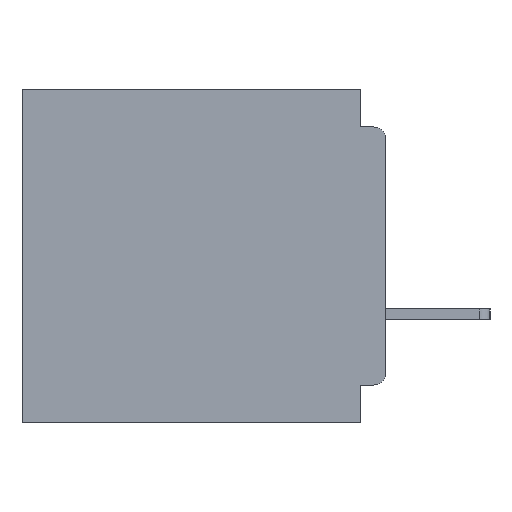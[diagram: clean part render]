
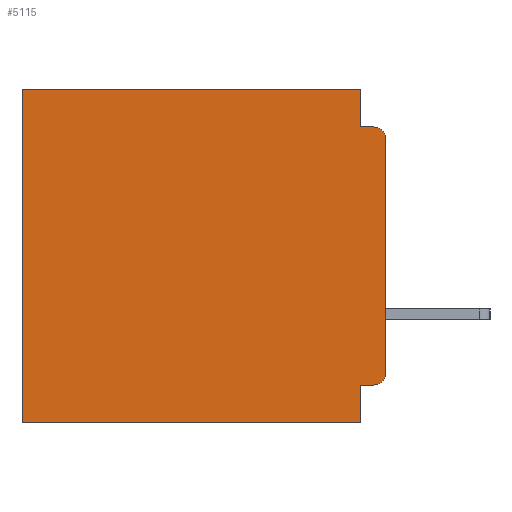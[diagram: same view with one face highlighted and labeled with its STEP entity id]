
A CAD part, left-side view. The second image highlights one B-rep face of the part: STEP entity #5115.
In plain terms, the highlighted planar face has unit normal (-1, 0, 0).
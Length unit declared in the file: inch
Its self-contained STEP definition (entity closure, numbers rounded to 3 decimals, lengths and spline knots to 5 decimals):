
#22 = LINE ( 'NONE', #43585, #37255 ) ;
#1250 = EDGE_CURVE ( 'NONE', #62377, #5661, #42428, .T. ) ;
#1425 = ORIENTED_EDGE ( 'NONE', *, *, #43986, .F. ) ;
#1690 = CARTESIAN_POINT ( 'NONE',  ( 0.3, 0.437, -0.4 ) ) ;
#2197 = CARTESIAN_POINT ( 'NONE',  ( 0.3, 0., -0.4 ) ) ;
#2217 = CARTESIAN_POINT ( 'NONE',  ( 0.3, 0., -0.355 ) ) ;
#5115 = ADVANCED_FACE ( 'NONE', ( #31455 ), #31283, .F. ) ;
#5163 = CIRCLE ( 'NONE', #60748, 0.015 ) ;
#5661 = VERTEX_POINT ( 'NONE', #1690 ) ;
#5747 = CARTESIAN_POINT ( 'NONE',  ( 0.3, 0.015, -0.06 ) ) ;
#5921 = VECTOR ( 'NONE', #22734, 39.37008 ) ;
#5989 = ORIENTED_EDGE ( 'NONE', *, *, #25638, .F. ) ;
#6560 = VERTEX_POINT ( 'NONE', #57812 ) ;
#6705 = DIRECTION ( 'NONE',  ( -1., 0., 0. ) ) ;
#7070 = DIRECTION ( 'NONE',  ( 1., 0., 0. ) ) ;
#9063 = VERTEX_POINT ( 'NONE', #48543 ) ;
#9723 = DIRECTION ( 'NONE',  ( 0., 0., -1. ) ) ;
#9816 = CARTESIAN_POINT ( 'NONE',  ( 0.3, 0.031, -0.4 ) ) ;
#9836 = VERTEX_POINT ( 'NONE', #16102 ) ;
#10659 = DIRECTION ( 'NONE',  ( 0., 0., -1. ) ) ;
#10803 = LINE ( 'NONE', #21135, #36539 ) ;
#12508 = VERTEX_POINT ( 'NONE', #9816 ) ;
#13091 = CARTESIAN_POINT ( 'NONE',  ( 0.3, 0.031, -0.4 ) ) ;
#13799 = LINE ( 'NONE', #33383, #52346 ) ;
#14125 = EDGE_CURVE ( 'NONE', #22895, #6560, #31922, .T. ) ;
#15956 = ORIENTED_EDGE ( 'NONE', *, *, #57442, .F. ) ;
#15957 = CARTESIAN_POINT ( 'NONE',  ( 0.3, 0.031, -0.355 ) ) ;
#16102 = CARTESIAN_POINT ( 'NONE',  ( 0.3, 0.015, -0.355 ) ) ;
#18170 = EDGE_CURVE ( 'NONE', #6560, #48201, #10803, .T. ) ;
#18197 = ORIENTED_EDGE ( 'NONE', *, *, #14125, .F. ) ;
#19009 = CARTESIAN_POINT ( 'NONE',  ( 0.3, 0.031, 0. ) ) ;
#19772 = AXIS2_PLACEMENT_3D ( 'NONE', #2197, #7070, #40961 ) ;
#21135 = CARTESIAN_POINT ( 'NONE',  ( 0.3, 0., -0.045 ) ) ;
#22161 = LINE ( 'NONE', #2217, #46366 ) ;
#22734 = DIRECTION ( 'NONE',  ( 0., 1., 0. ) ) ;
#22895 = VERTEX_POINT ( 'NONE', #56652 ) ;
#23789 = CARTESIAN_POINT ( 'NONE',  ( 0.3, 0.437, -0.4 ) ) ;
#24205 = ORIENTED_EDGE ( 'NONE', *, *, #62770, .F. ) ;
#25397 = VERTEX_POINT ( 'NONE', #54737 ) ;
#25561 = AXIS2_PLACEMENT_3D ( 'NONE', #35741, #6705, #40599 ) ;
#25638 = EDGE_CURVE ( 'NONE', #58649, #12508, #27592, .T. ) ;
#27592 = LINE ( 'NONE', #13091, #41976 ) ;
#27611 = CARTESIAN_POINT ( 'NONE',  ( 0.3, 0., 0. ) ) ;
#31283 = PLANE ( 'NONE',  #19772 ) ;
#31455 = FACE_OUTER_BOUND ( 'NONE', #59836, .T. ) ;
#31922 = LINE ( 'NONE', #19009, #56004 ) ;
#33383 = CARTESIAN_POINT ( 'NONE',  ( 0.3, 0., -0.4 ) ) ;
#35741 = CARTESIAN_POINT ( 'NONE',  ( 0.3, 0.015, -0.34 ) ) ;
#36539 = VECTOR ( 'NONE', #45273, 39.37008 ) ;
#37255 = VECTOR ( 'NONE', #9723, 39.37008 ) ;
#39030 = DIRECTION ( 'NONE',  ( 0., 0., -1. ) ) ;
#39647 = DIRECTION ( 'NONE',  ( -1., 0., 0. ) ) ;
#40599 = DIRECTION ( 'NONE',  ( 0., 0., -1. ) ) ;
#40961 = DIRECTION ( 'NONE',  ( 0., 0., -1. ) ) ;
#40986 = DIRECTION ( 'NONE',  ( 0., 1., 0. ) ) ;
#41264 = ORIENTED_EDGE ( 'NONE', *, *, #53343, .T. ) ;
#41976 = VECTOR ( 'NONE', #46914, 39.37008 ) ;
#42428 = LINE ( 'NONE', #23789, #53720 ) ;
#43585 = CARTESIAN_POINT ( 'NONE',  ( 0.3, 0., -0.4 ) ) ;
#43986 = EDGE_CURVE ( 'NONE', #9836, #58649, #22161, .T. ) ;
#45107 = CARTESIAN_POINT ( 'NONE',  ( 0.3, 0.437, 0. ) ) ;
#45195 = CARTESIAN_POINT ( 'NONE',  ( 0.3, 0.015, -0.045 ) ) ;
#45273 = DIRECTION ( 'NONE',  ( 0., -1., 0. ) ) ;
#46366 = VECTOR ( 'NONE', #40986, 39.37008 ) ;
#46914 = DIRECTION ( 'NONE',  ( 0., 0., -1. ) ) ;
#47483 = ORIENTED_EDGE ( 'NONE', *, *, #1250, .T. ) ;
#47508 = ORIENTED_EDGE ( 'NONE', *, *, #18170, .F. ) ;
#47730 = EDGE_CURVE ( 'NONE', #9836, #25397, #53389, .T. ) ;
#48201 = VERTEX_POINT ( 'NONE', #45195 ) ;
#48543 = CARTESIAN_POINT ( 'NONE',  ( 0.3, 0., -0.06 ) ) ;
#48696 = EDGE_CURVE ( 'NONE', #9063, #48201, #5163, .T. ) ;
#52346 = VECTOR ( 'NONE', #62223, 39.37008 ) ;
#53343 = EDGE_CURVE ( 'NONE', #22895, #62377, #58842, .T. ) ;
#53389 = CIRCLE ( 'NONE', #25561, 0.015 ) ;
#53720 = VECTOR ( 'NONE', #39030, 39.37008 ) ;
#54274 = ORIENTED_EDGE ( 'NONE', *, *, #48696, .T. ) ;
#54737 = CARTESIAN_POINT ( 'NONE',  ( 0.3, 0., -0.34 ) ) ;
#56004 = VECTOR ( 'NONE', #57596, 39.37008 ) ;
#56652 = CARTESIAN_POINT ( 'NONE',  ( 0.3, 0.031, 0. ) ) ;
#57442 = EDGE_CURVE ( 'NONE', #12508, #5661, #13799, .T. ) ;
#57596 = DIRECTION ( 'NONE',  ( 0., 0., -1. ) ) ;
#57812 = CARTESIAN_POINT ( 'NONE',  ( 0.3, 0.031, -0.045 ) ) ;
#58649 = VERTEX_POINT ( 'NONE', #15957 ) ;
#58842 = LINE ( 'NONE', #27611, #5921 ) ;
#59836 = EDGE_LOOP ( 'NONE', ( #24205, #54274, #47508, #18197, #41264, #47483, #15956, #5989, #1425, #62700 ) ) ;
#60748 = AXIS2_PLACEMENT_3D ( 'NONE', #5747, #39647, #10659 ) ;
#62223 = DIRECTION ( 'NONE',  ( 0., 1., 0. ) ) ;
#62377 = VERTEX_POINT ( 'NONE', #45107 ) ;
#62700 = ORIENTED_EDGE ( 'NONE', *, *, #47730, .T. ) ;
#62770 = EDGE_CURVE ( 'NONE', #9063, #25397, #22, .T. ) ;
